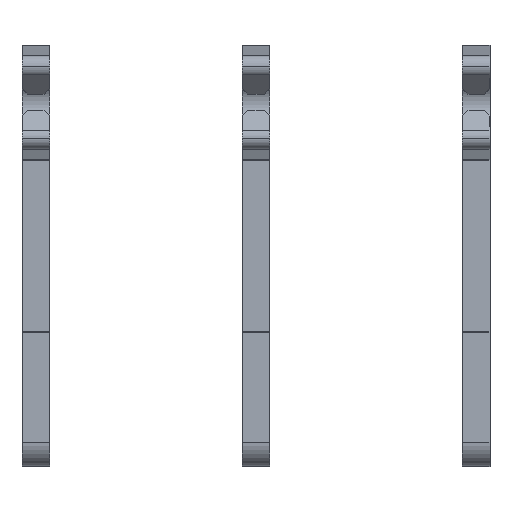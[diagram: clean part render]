
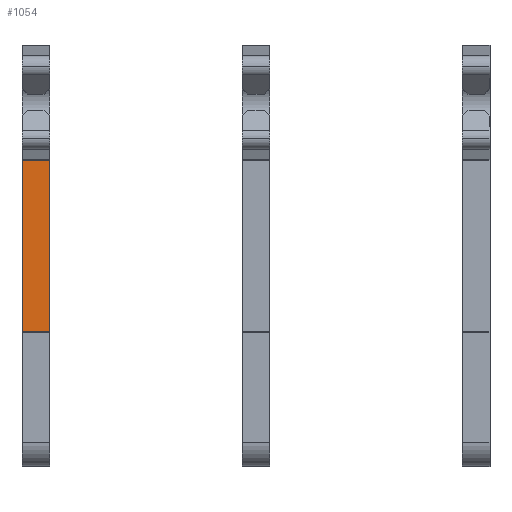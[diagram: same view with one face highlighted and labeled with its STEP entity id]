
A CAD part, top view. The second image highlights one B-rep face of the part: STEP entity #1054.
In plain terms, the highlighted planar face has unit normal (0, 0, 1).
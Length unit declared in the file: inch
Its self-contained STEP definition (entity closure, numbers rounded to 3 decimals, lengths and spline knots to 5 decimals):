
#13 = LINE ( 'NONE', #182, #1144 ) ;
#20 = EDGE_CURVE ( 'NONE', #1344, #194, #13, .T. ) ;
#39 = CARTESIAN_POINT ( 'NONE',  ( 0.0125, -0.208, -0.07 ) ) ;
#120 = DIRECTION ( 'NONE',  ( -1., 0., 0. ) ) ;
#182 = CARTESIAN_POINT ( 'NONE',  ( 0.0125, -0.208, -0.07 ) ) ;
#194 = VERTEX_POINT ( 'NONE', #769 ) ;
#201 = EDGE_CURVE ( 'NONE', #859, #1318, #319, .T. ) ;
#221 = EDGE_CURVE ( 'NONE', #859, #1344, #1390, .T. ) ;
#233 = ORIENTED_EDGE ( 'NONE', *, *, #221, .F. ) ;
#319 = LINE ( 'NONE', #674, #652 ) ;
#331 = DIRECTION ( 'NONE',  ( -1., 0., 0. ) ) ;
#367 = VECTOR ( 'NONE', #1124, 39.37008 ) ;
#605 = ORIENTED_EDGE ( 'NONE', *, *, #20, .F. ) ;
#618 = CARTESIAN_POINT ( 'NONE',  ( 0.0125, -0.052, -0.07 ) ) ;
#652 = VECTOR ( 'NONE', #120, 39.37008 ) ;
#669 = ORIENTED_EDGE ( 'NONE', *, *, #201, .T. ) ;
#674 = CARTESIAN_POINT ( 'NONE',  ( 0.0125, -0.052, -0.07 ) ) ;
#759 = PLANE ( 'NONE',  #1268 ) ;
#769 = CARTESIAN_POINT ( 'NONE',  ( -0.0125, -0.208, -0.07 ) ) ;
#859 = VERTEX_POINT ( 'NONE', #618 ) ;
#956 = DIRECTION ( 'NONE',  ( -1., 0., 0. ) ) ;
#1019 = EDGE_LOOP ( 'NONE', ( #1329, #605, #233, #669 ) ) ;
#1020 = CARTESIAN_POINT ( 'NONE',  ( -0.0125, -0.052, -0.07 ) ) ;
#1054 = ADVANCED_FACE ( 'NONE', ( #1393 ), #759, .F. ) ;
#1069 = DIRECTION ( 'NONE',  ( 0., 0., -1. ) ) ;
#1100 = DIRECTION ( 'NONE',  ( 0., -1., 0. ) ) ;
#1119 = CARTESIAN_POINT ( 'NONE',  ( -0.0125, -0.208, -0.07 ) ) ;
#1124 = DIRECTION ( 'NONE',  ( 0., -1., 0. ) ) ;
#1138 = LINE ( 'NONE', #1119, #367 ) ;
#1144 = VECTOR ( 'NONE', #956, 39.37008 ) ;
#1222 = CARTESIAN_POINT ( 'NONE',  ( 0.0125, -0.208, -0.07 ) ) ;
#1268 = AXIS2_PLACEMENT_3D ( 'NONE', #1290, #1069, #331 ) ;
#1270 = VECTOR ( 'NONE', #1100, 39.37008 ) ;
#1290 = CARTESIAN_POINT ( 'NONE',  ( 0.0125, -0.208, -0.07 ) ) ;
#1318 = VERTEX_POINT ( 'NONE', #1020 ) ;
#1329 = ORIENTED_EDGE ( 'NONE', *, *, #1346, .T. ) ;
#1344 = VERTEX_POINT ( 'NONE', #39 ) ;
#1346 = EDGE_CURVE ( 'NONE', #1318, #194, #1138, .T. ) ;
#1390 = LINE ( 'NONE', #1222, #1270 ) ;
#1393 = FACE_OUTER_BOUND ( 'NONE', #1019, .T. ) ;
